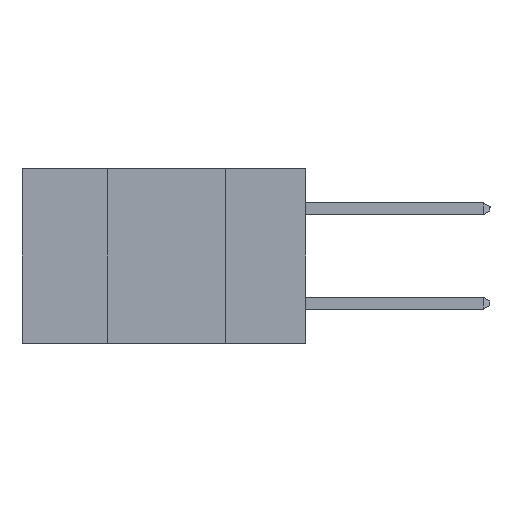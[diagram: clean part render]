
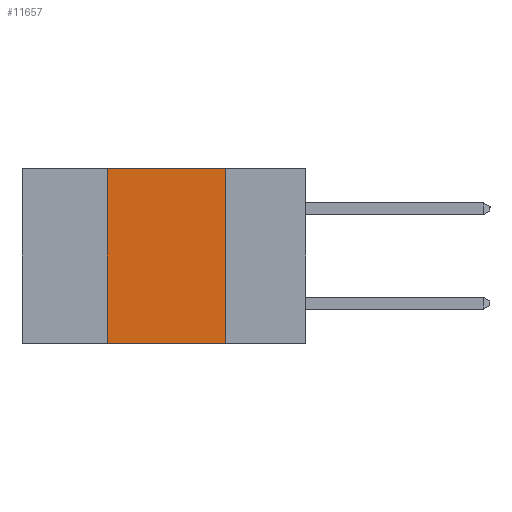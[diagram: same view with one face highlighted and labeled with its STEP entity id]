
A CAD part, left-side view. The second image highlights one B-rep face of the part: STEP entity #11657.
In plain terms, the highlighted planar face has unit normal (-1, 0, 0).
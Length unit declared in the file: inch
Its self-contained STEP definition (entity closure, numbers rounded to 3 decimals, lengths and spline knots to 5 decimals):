
#99 = PLANE ( 'NONE',  #3638 ) ;
#640 = VECTOR ( 'NONE', #14557, 39.37008 ) ;
#1177 = CARTESIAN_POINT ( 'NONE',  ( 0., 0.42, 0. ) ) ;
#1285 = EDGE_CURVE ( 'NONE', #10410, #6467, #4923, .T. ) ;
#2133 = LINE ( 'NONE', #10821, #3058 ) ;
#3058 = VECTOR ( 'NONE', #15926, 39.37008 ) ;
#3222 = CARTESIAN_POINT ( 'NONE',  ( 0., 0.42, -0.37 ) ) ;
#3638 = AXIS2_PLACEMENT_3D ( 'NONE', #12379, #8407, #12228 ) ;
#4459 = ORIENTED_EDGE ( 'NONE', *, *, #8677, .F. ) ;
#4656 = LINE ( 'NONE', #6038, #640 ) ;
#4923 = LINE ( 'NONE', #12620, #5331 ) ;
#5087 = EDGE_CURVE ( 'NONE', #15183, #6467, #4656, .T. ) ;
#5331 = VECTOR ( 'NONE', #9859, 39.37008 ) ;
#5654 = EDGE_LOOP ( 'NONE', ( #15550, #13881, #4459, #8623 ) ) ;
#6038 = CARTESIAN_POINT ( 'NONE',  ( 0., 0.6, -0.37 ) ) ;
#6083 = EDGE_CURVE ( 'NONE', #6436, #10410, #15173, .T. ) ;
#6436 = VERTEX_POINT ( 'NONE', #1177 ) ;
#6467 = VERTEX_POINT ( 'NONE', #12237 ) ;
#8407 = DIRECTION ( 'NONE',  ( 1., 0., 0. ) ) ;
#8623 = ORIENTED_EDGE ( 'NONE', *, *, #5087, .T. ) ;
#8645 = FACE_OUTER_BOUND ( 'NONE', #5654, .T. ) ;
#8677 = EDGE_CURVE ( 'NONE', #15183, #6436, #2133, .T. ) ;
#8761 = DIRECTION ( 'NONE',  ( 0., -1., 0. ) ) ;
#9859 = DIRECTION ( 'NONE',  ( 0., 0., -1. ) ) ;
#10410 = VERTEX_POINT ( 'NONE', #13680 ) ;
#10821 = CARTESIAN_POINT ( 'NONE',  ( 0., 0.42, -0.37 ) ) ;
#11355 = CARTESIAN_POINT ( 'NONE',  ( 0., 0.6, 0. ) ) ;
#11657 = ADVANCED_FACE ( 'NONE', ( #8645 ), #99, .F. ) ;
#11862 = VECTOR ( 'NONE', #8761, 39.37008 ) ;
#12228 = DIRECTION ( 'NONE',  ( 0., 0., -1. ) ) ;
#12237 = CARTESIAN_POINT ( 'NONE',  ( 0., 0.17, -0.37 ) ) ;
#12379 = CARTESIAN_POINT ( 'NONE',  ( 0., 0.6, 0. ) ) ;
#12620 = CARTESIAN_POINT ( 'NONE',  ( 0., 0.17, -0.37 ) ) ;
#13680 = CARTESIAN_POINT ( 'NONE',  ( 0., 0.17, 0. ) ) ;
#13881 = ORIENTED_EDGE ( 'NONE', *, *, #6083, .F. ) ;
#14557 = DIRECTION ( 'NONE',  ( 0., -1., 0. ) ) ;
#15173 = LINE ( 'NONE', #11355, #11862 ) ;
#15183 = VERTEX_POINT ( 'NONE', #3222 ) ;
#15550 = ORIENTED_EDGE ( 'NONE', *, *, #1285, .F. ) ;
#15926 = DIRECTION ( 'NONE',  ( 0., 0., 1. ) ) ;
